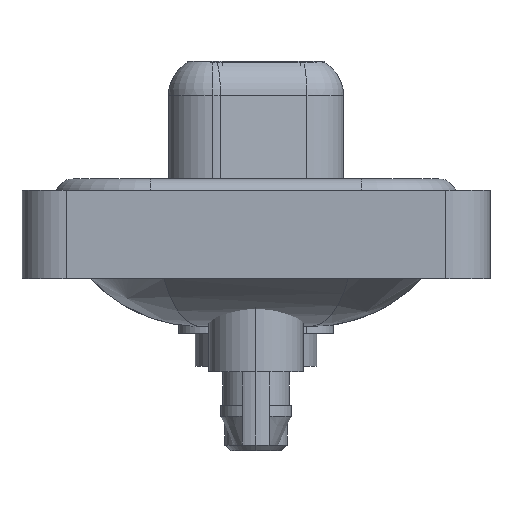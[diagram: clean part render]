
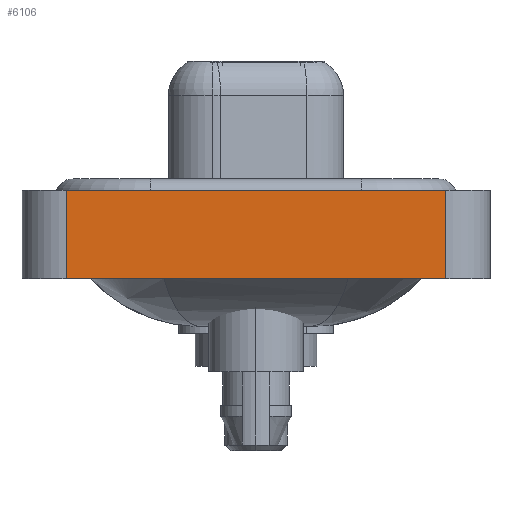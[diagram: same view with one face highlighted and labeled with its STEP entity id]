
A CAD part, left-side view. The second image highlights one B-rep face of the part: STEP entity #6106.
In plain terms, the highlighted planar face has unit normal (-1, 0, 0).
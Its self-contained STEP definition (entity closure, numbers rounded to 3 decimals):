
#261 = VECTOR ( 'NONE', #16158, 1000. ) ;
#366 = DIRECTION ( 'NONE',  ( 0., -1., 0. ) ) ;
#1008 = CARTESIAN_POINT ( 'NONE',  ( -7.3, -8.55, -3.6 ) ) ;
#2074 = DIRECTION ( 'NONE',  ( -1., 0., 0. ) ) ;
#2986 = EDGE_LOOP ( 'NONE', ( #10635, #9493, #11119, #7861 ) ) ;
#3200 = LINE ( 'NONE', #12576, #4591 ) ;
#3553 = CARTESIAN_POINT ( 'NONE',  ( -7.3, 8.55, 0.4 ) ) ;
#4591 = VECTOR ( 'NONE', #366, 1000. ) ;
#4598 = VECTOR ( 'NONE', #16377, 1000. ) ;
#4651 = FACE_OUTER_BOUND ( 'NONE', #2986, .T. ) ;
#6106 = ADVANCED_FACE ( 'NONE', ( #4651 ), #17188, .T. ) ;
#6428 = DIRECTION ( 'NONE',  ( 0., 0., 1. ) ) ;
#7861 = ORIENTED_EDGE ( 'NONE', *, *, #10263, .T. ) ;
#8688 = CARTESIAN_POINT ( 'NONE',  ( -7.3, -8.55, 0.4 ) ) ;
#8763 = VERTEX_POINT ( 'NONE', #3553 ) ;
#9493 = ORIENTED_EDGE ( 'NONE', *, *, #13470, .F. ) ;
#9497 = CARTESIAN_POINT ( 'NONE',  ( -7.3, -8.55, -3.6 ) ) ;
#10120 = CARTESIAN_POINT ( 'NONE',  ( -7.3, 8.55, -3.6 ) ) ;
#10263 = EDGE_CURVE ( 'NONE', #13142, #16727, #10851, .T. ) ;
#10635 = ORIENTED_EDGE ( 'NONE', *, *, #12276, .T. ) ;
#10716 = EDGE_CURVE ( 'NONE', #13142, #8763, #16794, .T. ) ;
#10851 = LINE ( 'NONE', #9497, #261 ) ;
#10983 = CARTESIAN_POINT ( 'NONE',  ( -7.3, -8.55, -3.6 ) ) ;
#11094 = VECTOR ( 'NONE', #15276, 1000. ) ;
#11119 = ORIENTED_EDGE ( 'NONE', *, *, #10716, .F. ) ;
#12276 = EDGE_CURVE ( 'NONE', #16727, #15708, #13386, .T. ) ;
#12576 = CARTESIAN_POINT ( 'NONE',  ( -7.3, -8.55, 0.4 ) ) ;
#13133 = AXIS2_PLACEMENT_3D ( 'NONE', #1008, #2074, #6428 ) ;
#13142 = VERTEX_POINT ( 'NONE', #17271 ) ;
#13386 = LINE ( 'NONE', #10983, #4598 ) ;
#13470 = EDGE_CURVE ( 'NONE', #8763, #15708, #3200, .T. ) ;
#14406 = CARTESIAN_POINT ( 'NONE',  ( -7.3, -8.55, -3.6 ) ) ;
#15276 = DIRECTION ( 'NONE',  ( 0., 0., 1. ) ) ;
#15708 = VERTEX_POINT ( 'NONE', #8688 ) ;
#16158 = DIRECTION ( 'NONE',  ( 0., -1., 0. ) ) ;
#16377 = DIRECTION ( 'NONE',  ( 0., 0., 1. ) ) ;
#16727 = VERTEX_POINT ( 'NONE', #14406 ) ;
#16794 = LINE ( 'NONE', #10120, #11094 ) ;
#17188 = PLANE ( 'NONE',  #13133 ) ;
#17271 = CARTESIAN_POINT ( 'NONE',  ( -7.3, 8.55, -3.6 ) ) ;
